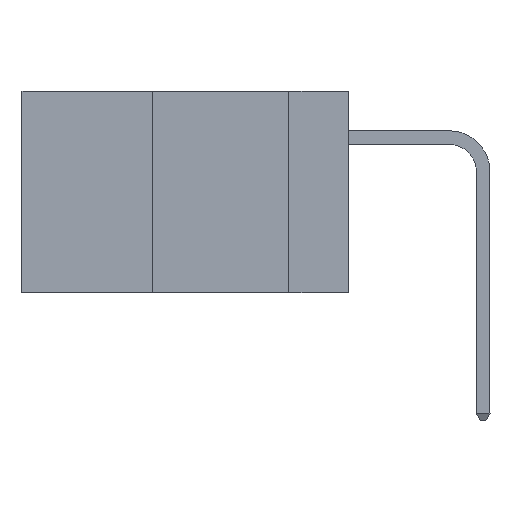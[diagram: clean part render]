
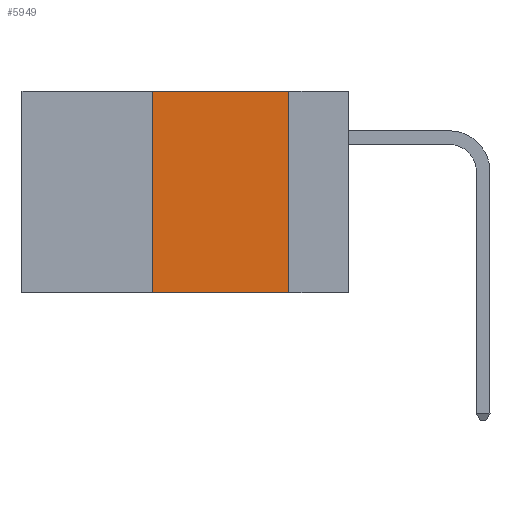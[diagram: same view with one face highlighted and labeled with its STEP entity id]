
A CAD part, left-side view. The second image highlights one B-rep face of the part: STEP entity #5949.
In plain terms, the highlighted planar face has unit normal (-1, 0, 0).
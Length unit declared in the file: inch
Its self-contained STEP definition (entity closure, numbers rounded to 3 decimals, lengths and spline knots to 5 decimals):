
#27 = ORIENTED_EDGE ( 'NONE', *, *, #7198, .F. ) ;
#750 = VERTEX_POINT ( 'NONE', #19701 ) ;
#1212 = CARTESIAN_POINT ( 'NONE',  ( 0., 0.11, 0. ) ) ;
#1982 = CARTESIAN_POINT ( 'NONE',  ( 0., 0.6, 0. ) ) ;
#3581 = CARTESIAN_POINT ( 'NONE',  ( 0., 0.6, 0. ) ) ;
#3666 = VERTEX_POINT ( 'NONE', #8591 ) ;
#3704 = FACE_OUTER_BOUND ( 'NONE', #5300, .T. ) ;
#3768 = DIRECTION ( 'NONE',  ( 0., -1., 0. ) ) ;
#4874 = VERTEX_POINT ( 'NONE', #16243 ) ;
#5012 = PLANE ( 'NONE',  #14777 ) ;
#5300 = EDGE_LOOP ( 'NONE', ( #9411, #27, #17657, #9952 ) ) ;
#5770 = VECTOR ( 'NONE', #3768, 39.37008 ) ;
#5949 = ADVANCED_FACE ( 'NONE', ( #3704 ), #5012, .F. ) ;
#7198 = EDGE_CURVE ( 'NONE', #9436, #4874, #9316, .T. ) ;
#7313 = EDGE_CURVE ( 'NONE', #3666, #750, #19139, .T. ) ;
#8591 = CARTESIAN_POINT ( 'NONE',  ( 0., 0.36, -0.37 ) ) ;
#8891 = LINE ( 'NONE', #1212, #18905 ) ;
#9193 = DIRECTION ( 'NONE',  ( 0., 0., -1. ) ) ;
#9316 = LINE ( 'NONE', #3581, #16370 ) ;
#9411 = ORIENTED_EDGE ( 'NONE', *, *, #16151, .F. ) ;
#9436 = VERTEX_POINT ( 'NONE', #17100 ) ;
#9952 = ORIENTED_EDGE ( 'NONE', *, *, #7313, .T. ) ;
#10926 = DIRECTION ( 'NONE',  ( 0., -1., 0. ) ) ;
#13150 = LINE ( 'NONE', #14740, #17056 ) ;
#14740 = CARTESIAN_POINT ( 'NONE',  ( 0., 0.36, 0. ) ) ;
#14777 = AXIS2_PLACEMENT_3D ( 'NONE', #1982, #18976, #17169 ) ;
#16063 = DIRECTION ( 'NONE',  ( 0., 0., 1. ) ) ;
#16151 = EDGE_CURVE ( 'NONE', #4874, #750, #8891, .T. ) ;
#16243 = CARTESIAN_POINT ( 'NONE',  ( 0., 0.11, 0. ) ) ;
#16370 = VECTOR ( 'NONE', #10926, 39.37008 ) ;
#17056 = VECTOR ( 'NONE', #16063, 39.37008 ) ;
#17100 = CARTESIAN_POINT ( 'NONE',  ( 0., 0.36, 0. ) ) ;
#17169 = DIRECTION ( 'NONE',  ( 0., 0., -1. ) ) ;
#17657 = ORIENTED_EDGE ( 'NONE', *, *, #18669, .F. ) ;
#18669 = EDGE_CURVE ( 'NONE', #3666, #9436, #13150, .T. ) ;
#18905 = VECTOR ( 'NONE', #9193, 39.37008 ) ;
#18976 = DIRECTION ( 'NONE',  ( 1., 0., 0. ) ) ;
#19139 = LINE ( 'NONE', #19241, #5770 ) ;
#19241 = CARTESIAN_POINT ( 'NONE',  ( 0., 0.6, -0.37 ) ) ;
#19701 = CARTESIAN_POINT ( 'NONE',  ( 0., 0.11, -0.37 ) ) ;
